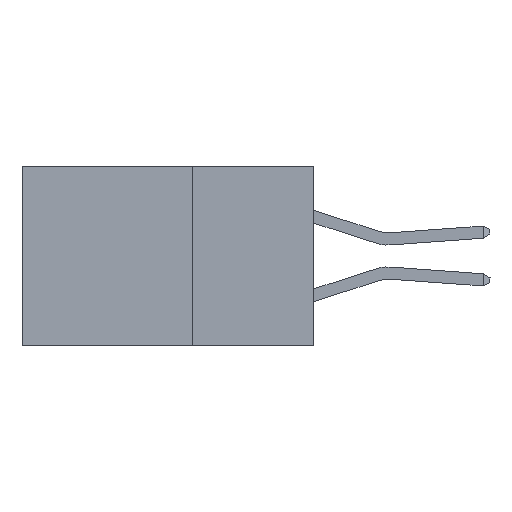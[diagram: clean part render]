
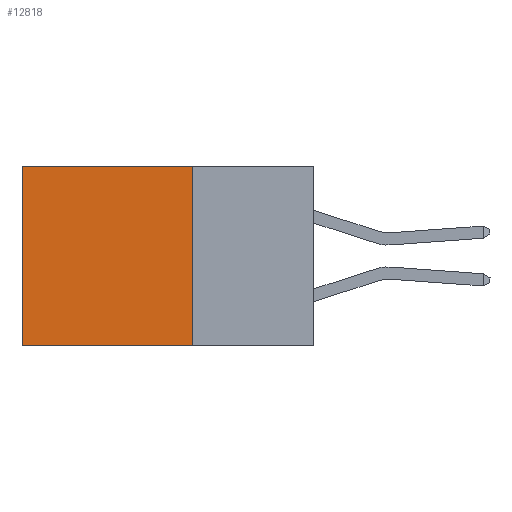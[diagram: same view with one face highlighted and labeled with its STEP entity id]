
A CAD part, left-side view. The second image highlights one B-rep face of the part: STEP entity #12818.
In plain terms, the highlighted planar face has unit normal (-1, 0, 0).
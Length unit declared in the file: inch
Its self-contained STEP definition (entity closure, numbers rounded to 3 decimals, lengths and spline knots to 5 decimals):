
#41 = VECTOR ( 'NONE', #8682, 39.37008 ) ;
#136 = LINE ( 'NONE', #6094, #15371 ) ;
#1934 = EDGE_CURVE ( 'NONE', #12808, #17221, #4033, .T. ) ;
#3257 = EDGE_CURVE ( 'NONE', #16787, #18943, #8835, .T. ) ;
#3391 = VECTOR ( 'NONE', #8565, 39.37008 ) ;
#4033 = LINE ( 'NONE', #4443, #12700 ) ;
#4298 = AXIS2_PLACEMENT_3D ( 'NONE', #9271, #5648, #18499 ) ;
#4443 = CARTESIAN_POINT ( 'NONE',  ( 0.2875, 0.25, 0. ) ) ;
#5436 = FACE_OUTER_BOUND ( 'NONE', #21707, .T. ) ;
#5474 = LINE ( 'NONE', #6847, #41 ) ;
#5648 = DIRECTION ( 'NONE',  ( 1., 0., 0. ) ) ;
#6094 = CARTESIAN_POINT ( 'NONE',  ( 0.2875, 0.25, 0. ) ) ;
#6294 = DIRECTION ( 'NONE',  ( 0., 1., 0. ) ) ;
#6847 = CARTESIAN_POINT ( 'NONE',  ( 0.2875, 0.6, 0. ) ) ;
#8057 = ORIENTED_EDGE ( 'NONE', *, *, #17941, .F. ) ;
#8565 = DIRECTION ( 'NONE',  ( 0., 1., 0. ) ) ;
#8682 = DIRECTION ( 'NONE',  ( 0., 0., -1. ) ) ;
#8762 = ORIENTED_EDGE ( 'NONE', *, *, #11243, .T. ) ;
#8835 = LINE ( 'NONE', #14087, #3391 ) ;
#9271 = CARTESIAN_POINT ( 'NONE',  ( 0.2875, 0.25, 0. ) ) ;
#11243 = EDGE_CURVE ( 'NONE', #17221, #18943, #5474, .T. ) ;
#12606 = CARTESIAN_POINT ( 'NONE',  ( 0.2875, 0.6, -0.37 ) ) ;
#12700 = VECTOR ( 'NONE', #6294, 39.37008 ) ;
#12808 = VERTEX_POINT ( 'NONE', #18426 ) ;
#12818 = ADVANCED_FACE ( 'NONE', ( #5436 ), #12954, .F. ) ;
#12954 = PLANE ( 'NONE',  #4298 ) ;
#13464 = DIRECTION ( 'NONE',  ( 0., 0., -1. ) ) ;
#13512 = CARTESIAN_POINT ( 'NONE',  ( 0.2875, 0.25, -0.37 ) ) ;
#13575 = ORIENTED_EDGE ( 'NONE', *, *, #3257, .F. ) ;
#14087 = CARTESIAN_POINT ( 'NONE',  ( 0.2875, 0.25, -0.37 ) ) ;
#15371 = VECTOR ( 'NONE', #13464, 39.37008 ) ;
#16787 = VERTEX_POINT ( 'NONE', #13512 ) ;
#17221 = VERTEX_POINT ( 'NONE', #21914 ) ;
#17779 = ORIENTED_EDGE ( 'NONE', *, *, #1934, .T. ) ;
#17941 = EDGE_CURVE ( 'NONE', #12808, #16787, #136, .T. ) ;
#18426 = CARTESIAN_POINT ( 'NONE',  ( 0.2875, 0.25, 0. ) ) ;
#18499 = DIRECTION ( 'NONE',  ( 0., 0., -1. ) ) ;
#18943 = VERTEX_POINT ( 'NONE', #12606 ) ;
#21707 = EDGE_LOOP ( 'NONE', ( #8762, #13575, #8057, #17779 ) ) ;
#21914 = CARTESIAN_POINT ( 'NONE',  ( 0.2875, 0.6, 0. ) ) ;
